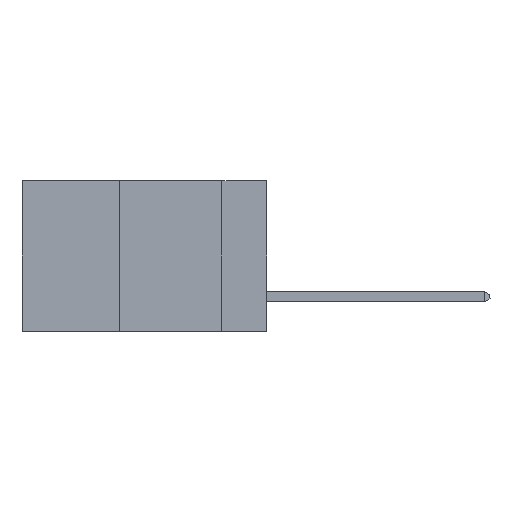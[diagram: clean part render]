
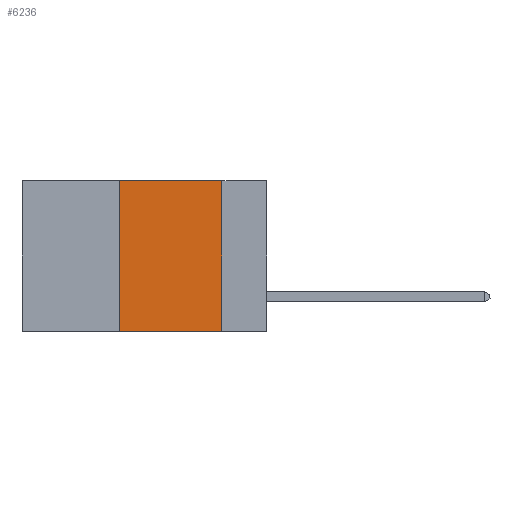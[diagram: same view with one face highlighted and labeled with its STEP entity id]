
A CAD part, left-side view. The second image highlights one B-rep face of the part: STEP entity #6236.
In plain terms, the highlighted planar face has unit normal (-1, 0, 0).
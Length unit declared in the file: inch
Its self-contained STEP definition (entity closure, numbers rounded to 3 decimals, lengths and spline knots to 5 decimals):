
#478 = VERTEX_POINT ( 'NONE', #6703 ) ;
#1436 = ORIENTED_EDGE ( 'NONE', *, *, #15304, .F. ) ;
#1964 = CARTESIAN_POINT ( 'NONE',  ( 0., 0.11, 0. ) ) ;
#2007 = ORIENTED_EDGE ( 'NONE', *, *, #15027, .F. ) ;
#2019 = DIRECTION ( 'NONE',  ( 0., 0., 1. ) ) ;
#2199 = VERTEX_POINT ( 'NONE', #19111 ) ;
#3302 = LINE ( 'NONE', #1964, #12913 ) ;
#3459 = DIRECTION ( 'NONE',  ( 0., -1., 0. ) ) ;
#5102 = PLANE ( 'NONE',  #5683 ) ;
#5683 = AXIS2_PLACEMENT_3D ( 'NONE', #17612, #19336, #8738 ) ;
#6236 = ADVANCED_FACE ( 'NONE', ( #7435 ), #5102, .F. ) ;
#6703 = CARTESIAN_POINT ( 'NONE',  ( 0., 0.11, -0.37 ) ) ;
#7235 = EDGE_LOOP ( 'NONE', ( #1436, #2007, #20982, #16974 ) ) ;
#7435 = FACE_OUTER_BOUND ( 'NONE', #7235, .T. ) ;
#7493 = CARTESIAN_POINT ( 'NONE',  ( 0., 0.36, 0. ) ) ;
#7563 = CARTESIAN_POINT ( 'NONE',  ( 0., 0.11, 0. ) ) ;
#8382 = EDGE_CURVE ( 'NONE', #2199, #478, #10097, .T. ) ;
#8472 = CARTESIAN_POINT ( 'NONE',  ( 0., 0.6, 0. ) ) ;
#8738 = DIRECTION ( 'NONE',  ( 0., 0., -1. ) ) ;
#8855 = CARTESIAN_POINT ( 'NONE',  ( 0., 0.6, -0.37 ) ) ;
#10097 = LINE ( 'NONE', #8855, #13791 ) ;
#10337 = CARTESIAN_POINT ( 'NONE',  ( 0., 0.36, 0. ) ) ;
#10532 = LINE ( 'NONE', #7493, #14216 ) ;
#11535 = EDGE_CURVE ( 'NONE', #2199, #11920, #10532, .T. ) ;
#11920 = VERTEX_POINT ( 'NONE', #10337 ) ;
#12913 = VECTOR ( 'NONE', #14667, 39.37008 ) ;
#13791 = VECTOR ( 'NONE', #3459, 39.37008 ) ;
#14216 = VECTOR ( 'NONE', #2019, 39.37008 ) ;
#14340 = VECTOR ( 'NONE', #15692, 39.37008 ) ;
#14667 = DIRECTION ( 'NONE',  ( 0., 0., -1. ) ) ;
#15027 = EDGE_CURVE ( 'NONE', #11920, #15708, #18978, .T. ) ;
#15304 = EDGE_CURVE ( 'NONE', #15708, #478, #3302, .T. ) ;
#15692 = DIRECTION ( 'NONE',  ( 0., -1., 0. ) ) ;
#15708 = VERTEX_POINT ( 'NONE', #7563 ) ;
#16974 = ORIENTED_EDGE ( 'NONE', *, *, #8382, .T. ) ;
#17612 = CARTESIAN_POINT ( 'NONE',  ( 0., 0.6, 0. ) ) ;
#18978 = LINE ( 'NONE', #8472, #14340 ) ;
#19111 = CARTESIAN_POINT ( 'NONE',  ( 0., 0.36, -0.37 ) ) ;
#19336 = DIRECTION ( 'NONE',  ( 1., 0., 0. ) ) ;
#20982 = ORIENTED_EDGE ( 'NONE', *, *, #11535, .F. ) ;
